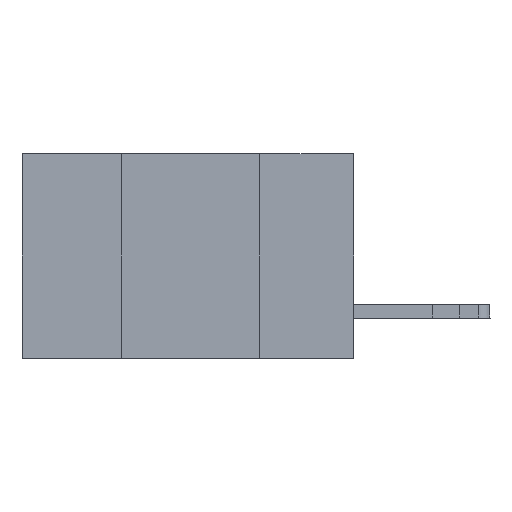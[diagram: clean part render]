
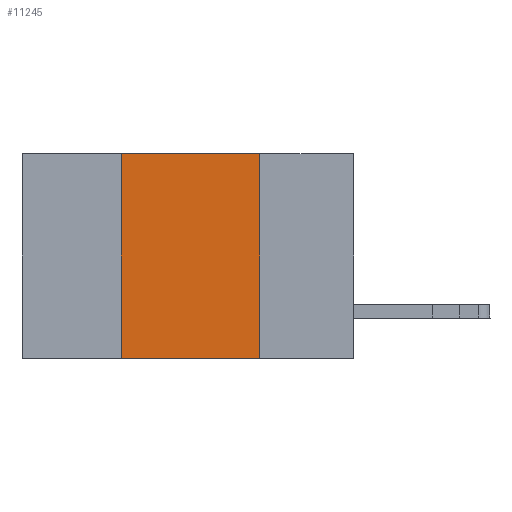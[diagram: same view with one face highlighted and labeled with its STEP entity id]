
A CAD part, left-side view. The second image highlights one B-rep face of the part: STEP entity #11245.
In plain terms, the highlighted planar face has unit normal (-1, 0, 0).
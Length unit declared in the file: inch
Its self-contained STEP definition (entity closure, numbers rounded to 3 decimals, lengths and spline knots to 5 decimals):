
#222 = EDGE_CURVE ( 'NONE', #32639, #20774, #14221, .T. ) ;
#573 = CARTESIAN_POINT ( 'NONE',  ( 0., 0.42, 0. ) ) ;
#768 = CARTESIAN_POINT ( 'NONE',  ( 0., 0.42, 0. ) ) ;
#854 = VECTOR ( 'NONE', #25125, 39.37008 ) ;
#1745 = AXIS2_PLACEMENT_3D ( 'NONE', #10409, #13152, #21419 ) ;
#2412 = CARTESIAN_POINT ( 'NONE',  ( 0., 0.6, 0. ) ) ;
#7450 = LINE ( 'NONE', #2412, #15135 ) ;
#7914 = PLANE ( 'NONE',  #1745 ) ;
#9149 = CARTESIAN_POINT ( 'NONE',  ( 0., 0.17, 0. ) ) ;
#9930 = EDGE_CURVE ( 'NONE', #20789, #32639, #7450, .T. ) ;
#10409 = CARTESIAN_POINT ( 'NONE',  ( 0., 0.6, 0. ) ) ;
#10825 = DIRECTION ( 'NONE',  ( 0., -1., 0. ) ) ;
#11245 = ADVANCED_FACE ( 'NONE', ( #26596 ), #7914, .F. ) ;
#11715 = ORIENTED_EDGE ( 'NONE', *, *, #222, .F. ) ;
#12705 = CARTESIAN_POINT ( 'NONE',  ( 0., 0.6, -0.37 ) ) ;
#13152 = DIRECTION ( 'NONE',  ( 1., 0., 0. ) ) ;
#14221 = LINE ( 'NONE', #9149, #35244 ) ;
#15135 = VECTOR ( 'NONE', #10825, 39.37008 ) ;
#16197 = DIRECTION ( 'NONE',  ( 0., 0., -1. ) ) ;
#16495 = ORIENTED_EDGE ( 'NONE', *, *, #9930, .F. ) ;
#16651 = CARTESIAN_POINT ( 'NONE',  ( 0., 0.42, -0.37 ) ) ;
#17353 = CARTESIAN_POINT ( 'NONE',  ( 0., 0.17, -0.37 ) ) ;
#19667 = DIRECTION ( 'NONE',  ( 0., 0., 1. ) ) ;
#20774 = VERTEX_POINT ( 'NONE', #17353 ) ;
#20789 = VERTEX_POINT ( 'NONE', #768 ) ;
#21352 = CARTESIAN_POINT ( 'NONE',  ( 0., 0.17, 0. ) ) ;
#21419 = DIRECTION ( 'NONE',  ( 0., 0., -1. ) ) ;
#21957 = EDGE_LOOP ( 'NONE', ( #11715, #16495, #23358, #26870 ) ) ;
#23358 = ORIENTED_EDGE ( 'NONE', *, *, #23490, .F. ) ;
#23490 = EDGE_CURVE ( 'NONE', #26898, #20789, #24933, .T. ) ;
#24933 = LINE ( 'NONE', #573, #31825 ) ;
#25125 = DIRECTION ( 'NONE',  ( 0., -1., 0. ) ) ;
#26510 = LINE ( 'NONE', #12705, #854 ) ;
#26596 = FACE_OUTER_BOUND ( 'NONE', #21957, .T. ) ;
#26870 = ORIENTED_EDGE ( 'NONE', *, *, #28296, .T. ) ;
#26898 = VERTEX_POINT ( 'NONE', #16651 ) ;
#28296 = EDGE_CURVE ( 'NONE', #26898, #20774, #26510, .T. ) ;
#31825 = VECTOR ( 'NONE', #19667, 39.37008 ) ;
#32639 = VERTEX_POINT ( 'NONE', #21352 ) ;
#35244 = VECTOR ( 'NONE', #16197, 39.37008 ) ;
